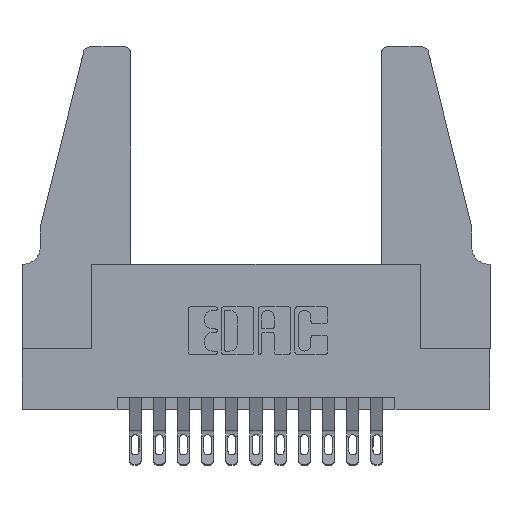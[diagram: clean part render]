
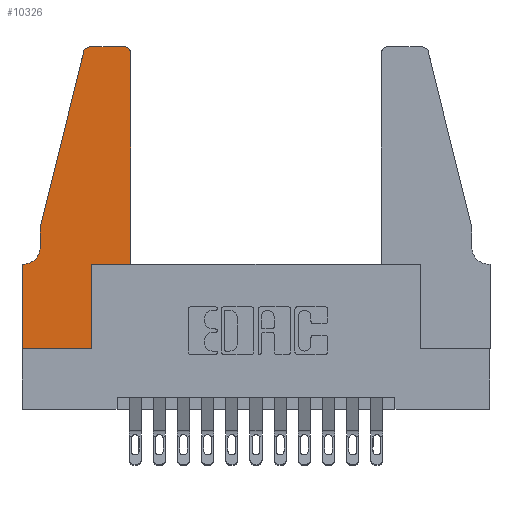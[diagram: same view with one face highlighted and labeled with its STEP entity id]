
A CAD part, top view. The second image highlights one B-rep face of the part: STEP entity #10326.
In plain terms, the highlighted planar face has unit normal (0, 0, 1).
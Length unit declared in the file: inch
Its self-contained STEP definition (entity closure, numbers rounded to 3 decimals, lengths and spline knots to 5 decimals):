
#71 = ORIENTED_EDGE ( 'NONE', *, *, #2003, .T. ) ;
#620 = ORIENTED_EDGE ( 'NONE', *, *, #5725, .T. ) ;
#758 = VECTOR ( 'NONE', #6440, 39.37008 ) ;
#995 = CARTESIAN_POINT ( 'NONE',  ( 0.4505, 1.22, 0.37 ) ) ;
#1091 = VERTEX_POINT ( 'NONE', #10091 ) ;
#1200 = CARTESIAN_POINT ( 'NONE',  ( 0., 0., 0.37 ) ) ;
#1247 = VERTEX_POINT ( 'NONE', #6518 ) ;
#1255 = CIRCLE ( 'NONE', #14115, 0.03 ) ;
#1270 = EDGE_CURVE ( 'NONE', #3173, #1377, #5362, .T. ) ;
#1332 = VERTEX_POINT ( 'NONE', #11830 ) ;
#1353 = VECTOR ( 'NONE', #8427, 39.37008 ) ;
#1377 = VERTEX_POINT ( 'NONE', #14118 ) ;
#1626 = AXIS2_PLACEMENT_3D ( 'NONE', #3533, #15248, #10609 ) ;
#1796 = DIRECTION ( 'NONE',  ( -1., 0., 0. ) ) ;
#1875 = CARTESIAN_POINT ( 'NONE',  ( 0., 0., 0.37 ) ) ;
#2003 = EDGE_CURVE ( 'NONE', #3282, #3173, #14216, .T. ) ;
#2088 = ORIENTED_EDGE ( 'NONE', *, *, #9761, .T. ) ;
#2499 = CARTESIAN_POINT ( 'NONE',  ( 0.4505, 0.35, 0.37 ) ) ;
#2941 = VECTOR ( 'NONE', #10331, 39.37008 ) ;
#3159 = EDGE_CURVE ( 'NONE', #12547, #1091, #1255, .T. ) ;
#3173 = VERTEX_POINT ( 'NONE', #995 ) ;
#3282 = VERTEX_POINT ( 'NONE', #2499 ) ;
#3287 = AXIS2_PLACEMENT_3D ( 'NONE', #9247, #15225, #3449 ) ;
#3449 = DIRECTION ( 'NONE',  ( 1., 0., 0. ) ) ;
#3456 = CARTESIAN_POINT ( 'NONE',  ( 0.4505, 0.35, 0.37 ) ) ;
#3476 = VECTOR ( 'NONE', #13609, 39.37008 ) ;
#3512 = CARTESIAN_POINT ( 'NONE',  ( 0.0755, 0.5, 0.37 ) ) ;
#3524 = VERTEX_POINT ( 'NONE', #13840 ) ;
#3533 = CARTESIAN_POINT ( 'NONE',  ( 0.4205, 1.22, 0.37 ) ) ;
#3677 = VECTOR ( 'NONE', #1796, 39.37008 ) ;
#3828 = CARTESIAN_POINT ( 'NONE',  ( 0.0755, 0.5, 0.37 ) ) ;
#3836 = CARTESIAN_POINT ( 'NONE',  ( 0., 0., 0.37 ) ) ;
#3874 = VECTOR ( 'NONE', #12911, 39.37008 ) ;
#4297 = EDGE_CURVE ( 'NONE', #8679, #3282, #11979, .T. ) ;
#4604 = DIRECTION ( 'NONE',  ( 0., 0., -1. ) ) ;
#4847 = VECTOR ( 'NONE', #5842, 39.37008 ) ;
#5011 = DIRECTION ( 'NONE',  ( -1., 0., 0. ) ) ;
#5362 = CIRCLE ( 'NONE', #1626, 0.03 ) ;
#5455 = CARTESIAN_POINT ( 'NONE',  ( 0.2865, 0.35, 0.37 ) ) ;
#5592 = CARTESIAN_POINT ( 'NONE',  ( 0.0755, 0.5, 0.37 ) ) ;
#5725 = EDGE_CURVE ( 'NONE', #1377, #12547, #13431, .T. ) ;
#5842 = DIRECTION ( 'NONE',  ( 0., -1., 0. ) ) ;
#6440 = DIRECTION ( 'NONE',  ( 1., 0., 0. ) ) ;
#6518 = CARTESIAN_POINT ( 'NONE',  ( 0.0755, 0.42, 0.37 ) ) ;
#6609 = VERTEX_POINT ( 'NONE', #3512 ) ;
#6825 = EDGE_CURVE ( 'NONE', #1091, #6609, #14680, .T. ) ;
#6966 = ORIENTED_EDGE ( 'NONE', *, *, #13144, .T. ) ;
#7002 = CARTESIAN_POINT ( 'NONE',  ( 0.2605, 1.25, 0.37 ) ) ;
#7134 = VECTOR ( 'NONE', #11517, 39.37008 ) ;
#7161 = CARTESIAN_POINT ( 'NONE',  ( 0.2865, 0.35, 0.37 ) ) ;
#7640 = CARTESIAN_POINT ( 'NONE',  ( 0.4505, 0.35, 0.37 ) ) ;
#7670 = EDGE_CURVE ( 'NONE', #6609, #1247, #8595, .T. ) ;
#7873 = VECTOR ( 'NONE', #14456, 39.37008 ) ;
#7901 = EDGE_CURVE ( 'NONE', #3524, #8679, #11697, .T. ) ;
#8098 = DIRECTION ( 'NONE',  ( 0., 0., 1. ) ) ;
#8129 = LINE ( 'NONE', #1200, #3874 ) ;
#8427 = DIRECTION ( 'NONE',  ( 0., 1., 0. ) ) ;
#8595 = LINE ( 'NONE', #5592, #4847 ) ;
#8679 = VERTEX_POINT ( 'NONE', #5455 ) ;
#8747 = FACE_OUTER_BOUND ( 'NONE', #9143, .T. ) ;
#8760 = ORIENTED_EDGE ( 'NONE', *, *, #7901, .T. ) ;
#9100 = LINE ( 'NONE', #3836, #758 ) ;
#9143 = EDGE_LOOP ( 'NONE', ( #620, #14733, #10182, #15074, #10752, #6966, #2088, #14531, #8760, #14478, #71, #13279 ) ) ;
#9247 = CARTESIAN_POINT ( 'NONE',  ( 0., 0.35, 0.37 ) ) ;
#9424 = CIRCLE ( 'NONE', #11114, 0.07 ) ;
#9584 = CARTESIAN_POINT ( 'NONE',  ( 0.0055, 0.42, 0.37 ) ) ;
#9761 = EDGE_CURVE ( 'NONE', #13006, #11469, #8129, .T. ) ;
#9785 = EDGE_CURVE ( 'NONE', #1247, #1332, #9424, .T. ) ;
#10091 = CARTESIAN_POINT ( 'NONE',  ( 0.25487, 1.22718, 0.37 ) ) ;
#10182 = ORIENTED_EDGE ( 'NONE', *, *, #6825, .T. ) ;
#10326 = ADVANCED_FACE ( 'NONE', ( #8747 ), #12686, .T. ) ;
#10331 = DIRECTION ( 'NONE',  ( 0., 1., 0. ) ) ;
#10445 = EDGE_CURVE ( 'NONE', #11469, #3524, #9100, .T. ) ;
#10568 = DIRECTION ( 'NONE',  ( 1., 0., 0. ) ) ;
#10609 = DIRECTION ( 'NONE',  ( 1., 0., 0. ) ) ;
#10752 = ORIENTED_EDGE ( 'NONE', *, *, #9785, .T. ) ;
#11114 = AXIS2_PLACEMENT_3D ( 'NONE', #9584, #4604, #5011 ) ;
#11469 = VERTEX_POINT ( 'NONE', #1875 ) ;
#11517 = DIRECTION ( 'NONE',  ( -1., 0., 0. ) ) ;
#11697 = LINE ( 'NONE', #7161, #1353 ) ;
#11702 = CARTESIAN_POINT ( 'NONE',  ( 0.284, 1.22, 0.37 ) ) ;
#11830 = CARTESIAN_POINT ( 'NONE',  ( 0.0055, 0.35, 0.37 ) ) ;
#11979 = LINE ( 'NONE', #7640, #3476 ) ;
#12160 = LINE ( 'NONE', #12470, #3677 ) ;
#12470 = CARTESIAN_POINT ( 'NONE',  ( 0.0755, 0.35, 0.37 ) ) ;
#12547 = VERTEX_POINT ( 'NONE', #13216 ) ;
#12686 = PLANE ( 'NONE',  #3287 ) ;
#12911 = DIRECTION ( 'NONE',  ( 0., -1., 0. ) ) ;
#13006 = VERTEX_POINT ( 'NONE', #13383 ) ;
#13144 = EDGE_CURVE ( 'NONE', #1332, #13006, #12160, .T. ) ;
#13216 = CARTESIAN_POINT ( 'NONE',  ( 0.284, 1.25, 0.37 ) ) ;
#13279 = ORIENTED_EDGE ( 'NONE', *, *, #1270, .T. ) ;
#13383 = CARTESIAN_POINT ( 'NONE',  ( 0., 0.35, 0.37 ) ) ;
#13431 = LINE ( 'NONE', #7002, #7134 ) ;
#13609 = DIRECTION ( 'NONE',  ( 1., 0., 0. ) ) ;
#13840 = CARTESIAN_POINT ( 'NONE',  ( 0.2865, 0., 0.37 ) ) ;
#14115 = AXIS2_PLACEMENT_3D ( 'NONE', #11702, #8098, #10568 ) ;
#14118 = CARTESIAN_POINT ( 'NONE',  ( 0.4205, 1.25, 0.37 ) ) ;
#14216 = LINE ( 'NONE', #3456, #2941 ) ;
#14456 = DIRECTION ( 'NONE',  ( -0.239, -0.971, 0. ) ) ;
#14478 = ORIENTED_EDGE ( 'NONE', *, *, #4297, .T. ) ;
#14531 = ORIENTED_EDGE ( 'NONE', *, *, #10445, .T. ) ;
#14680 = LINE ( 'NONE', #3828, #7873 ) ;
#14733 = ORIENTED_EDGE ( 'NONE', *, *, #3159, .T. ) ;
#15074 = ORIENTED_EDGE ( 'NONE', *, *, #7670, .T. ) ;
#15225 = DIRECTION ( 'NONE',  ( 0., 0., 1. ) ) ;
#15248 = DIRECTION ( 'NONE',  ( 0., 0., 1. ) ) ;
